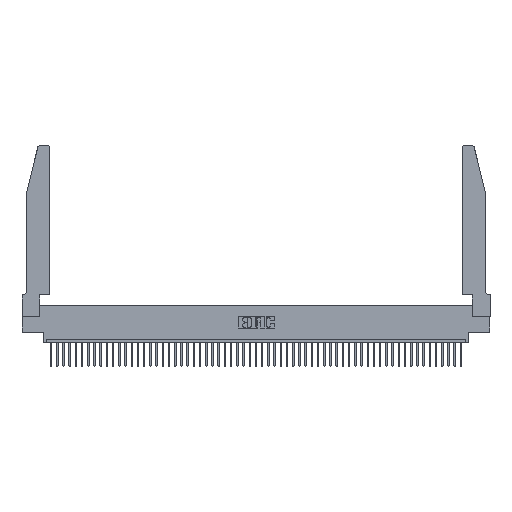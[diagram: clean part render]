
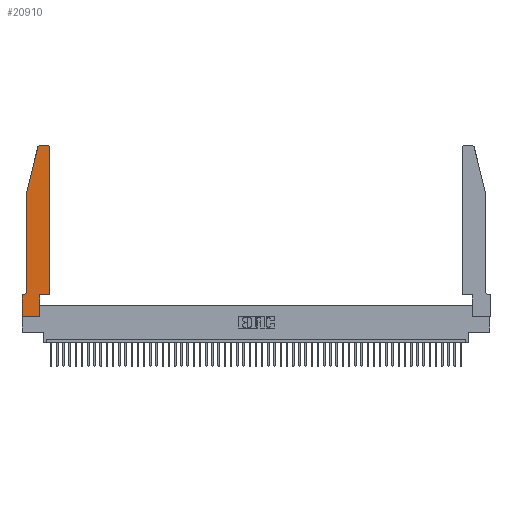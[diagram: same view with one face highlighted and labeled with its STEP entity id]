
A CAD part, top view. The second image highlights one B-rep face of the part: STEP entity #20910.
In plain terms, the highlighted planar face has unit normal (0, 0, 1).
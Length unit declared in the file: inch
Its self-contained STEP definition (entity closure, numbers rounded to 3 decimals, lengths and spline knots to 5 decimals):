
#106 = DIRECTION ( 'NONE',  ( 1., 0., 0. ) ) ;
#670 = CARTESIAN_POINT ( 'NONE',  ( 0.4505, 2.72, 0.37 ) ) ;
#976 = PLANE ( 'NONE',  #9480 ) ;
#1471 = VECTOR ( 'NONE', #15062, 39.37008 ) ;
#2574 = VECTOR ( 'NONE', #45254, 39.37008 ) ;
#3251 = CARTESIAN_POINT ( 'NONE',  ( 0.284, 2.72, 0.37 ) ) ;
#4625 = DIRECTION ( 'NONE',  ( -0.239, -0.971, 0. ) ) ;
#5099 = ORIENTED_EDGE ( 'NONE', *, *, #19223, .T. ) ;
#5565 = ORIENTED_EDGE ( 'NONE', *, *, #37497, .T. ) ;
#5788 = DIRECTION ( 'NONE',  ( -1., 0., 0. ) ) ;
#6047 = CARTESIAN_POINT ( 'NONE',  ( 0.0755, 0.42, 0.37 ) ) ;
#6204 = VERTEX_POINT ( 'NONE', #6047 ) ;
#6361 = VERTEX_POINT ( 'NONE', #27538 ) ;
#7352 = VERTEX_POINT ( 'NONE', #7887 ) ;
#7745 = CARTESIAN_POINT ( 'NONE',  ( 0.25487, 2.72718, 0.37 ) ) ;
#7887 = CARTESIAN_POINT ( 'NONE',  ( 0.0755, 2., 0.37 ) ) ;
#8169 = EDGE_CURVE ( 'NONE', #28078, #36773, #36141, .T. ) ;
#8439 = VECTOR ( 'NONE', #10460, 39.37008 ) ;
#9480 = AXIS2_PLACEMENT_3D ( 'NONE', #13320, #24859, #17191 ) ;
#9971 = DIRECTION ( 'NONE',  ( -1., 0., 0. ) ) ;
#10381 = VECTOR ( 'NONE', #5788, 39.37008 ) ;
#10450 = VERTEX_POINT ( 'NONE', #43552 ) ;
#10460 = DIRECTION ( 'NONE',  ( 0., -1., 0. ) ) ;
#10869 = VERTEX_POINT ( 'NONE', #31786 ) ;
#12723 = VECTOR ( 'NONE', #27065, 39.37008 ) ;
#12754 = CARTESIAN_POINT ( 'NONE',  ( 0.0755, 2., 0.37 ) ) ;
#12926 = CARTESIAN_POINT ( 'NONE',  ( 0.2865, 0.35, 0.37 ) ) ;
#13083 = EDGE_CURVE ( 'NONE', #6204, #28078, #36966, .T. ) ;
#13117 = ORIENTED_EDGE ( 'NONE', *, *, #24074, .T. ) ;
#13320 = CARTESIAN_POINT ( 'NONE',  ( 0., 0.35, 0.37 ) ) ;
#13763 = ORIENTED_EDGE ( 'NONE', *, *, #22768, .T. ) ;
#14435 = CARTESIAN_POINT ( 'NONE',  ( 0.0055, 0.35, 0.37 ) ) ;
#15062 = DIRECTION ( 'NONE',  ( 0., 1., 0. ) ) ;
#15123 = CARTESIAN_POINT ( 'NONE',  ( 0., 0.35, 0.37 ) ) ;
#15197 = LINE ( 'NONE', #22498, #2574 ) ;
#15308 = EDGE_CURVE ( 'NONE', #36773, #22337, #51869, .T. ) ;
#16344 = AXIS2_PLACEMENT_3D ( 'NONE', #20678, #28684, #21019 ) ;
#16410 = CARTESIAN_POINT ( 'NONE',  ( 0.4205, 2.72, 0.37 ) ) ;
#17191 = DIRECTION ( 'NONE',  ( 1., 0., 0. ) ) ;
#18412 = CARTESIAN_POINT ( 'NONE',  ( 0., 0., 0.37 ) ) ;
#19039 = CARTESIAN_POINT ( 'NONE',  ( 0.4505, 0.35, 0.37 ) ) ;
#19223 = EDGE_CURVE ( 'NONE', #10869, #6361, #35547, .T. ) ;
#20595 = EDGE_CURVE ( 'NONE', #28751, #26827, #34877, .T. ) ;
#20678 = CARTESIAN_POINT ( 'NONE',  ( 0.0055, 0.42, 0.37 ) ) ;
#20910 = ADVANCED_FACE ( 'NONE', ( #49197 ), #976, .T. ) ;
#21019 = DIRECTION ( 'NONE',  ( -1., 0., 0. ) ) ;
#21156 = VECTOR ( 'NONE', #4625, 39.37008 ) ;
#22337 = VERTEX_POINT ( 'NONE', #32782 ) ;
#22498 = CARTESIAN_POINT ( 'NONE',  ( 0.4505, 0.35, 0.37 ) ) ;
#22592 = DIRECTION ( 'NONE',  ( 0., -1., 0. ) ) ;
#22768 = EDGE_CURVE ( 'NONE', #7352, #6204, #40495, .T. ) ;
#23132 = VERTEX_POINT ( 'NONE', #670 ) ;
#23422 = LINE ( 'NONE', #19039, #12723 ) ;
#23601 = VECTOR ( 'NONE', #9971, 39.37008 ) ;
#23898 = CARTESIAN_POINT ( 'NONE',  ( 0.0755, 2., 0.37 ) ) ;
#24074 = EDGE_CURVE ( 'NONE', #10450, #23132, #23422, .T. ) ;
#24859 = DIRECTION ( 'NONE',  ( 0., 0., 1. ) ) ;
#24944 = EDGE_CURVE ( 'NONE', #26827, #10450, #15197, .T. ) ;
#25930 = CARTESIAN_POINT ( 'NONE',  ( 0.0755, 0.35, 0.37 ) ) ;
#26827 = VERTEX_POINT ( 'NONE', #12926 ) ;
#27065 = DIRECTION ( 'NONE',  ( 0., 1., 0. ) ) ;
#27412 = DIRECTION ( 'NONE',  ( 0., 0., 1. ) ) ;
#27538 = CARTESIAN_POINT ( 'NONE',  ( 0.284, 2.75, 0.37 ) ) ;
#28068 = CARTESIAN_POINT ( 'NONE',  ( 0., 0., 0.37 ) ) ;
#28078 = VERTEX_POINT ( 'NONE', #14435 ) ;
#28684 = DIRECTION ( 'NONE',  ( 0., 0., -1. ) ) ;
#28751 = VERTEX_POINT ( 'NONE', #45016 ) ;
#29571 = ORIENTED_EDGE ( 'NONE', *, *, #20595, .T. ) ;
#29642 = AXIS2_PLACEMENT_3D ( 'NONE', #16410, #48709, #106 ) ;
#30642 = AXIS2_PLACEMENT_3D ( 'NONE', #3251, #27412, #43130 ) ;
#31010 = EDGE_CURVE ( 'NONE', #6361, #39808, #44079, .T. ) ;
#31786 = CARTESIAN_POINT ( 'NONE',  ( 0.4205, 2.75, 0.37 ) ) ;
#32782 = CARTESIAN_POINT ( 'NONE',  ( 0., 0., 0.37 ) ) ;
#33013 = VECTOR ( 'NONE', #22592, 39.37008 ) ;
#34384 = EDGE_LOOP ( 'NONE', ( #5099, #35303, #5565, #13763, #36234, #51106, #35960, #47236, #29571, #40904, #13117, #43410 ) ) ;
#34877 = LINE ( 'NONE', #43309, #1471 ) ;
#35303 = ORIENTED_EDGE ( 'NONE', *, *, #31010, .T. ) ;
#35547 = LINE ( 'NONE', #49705, #10381 ) ;
#35960 = ORIENTED_EDGE ( 'NONE', *, *, #15308, .T. ) ;
#36141 = LINE ( 'NONE', #25930, #23601 ) ;
#36234 = ORIENTED_EDGE ( 'NONE', *, *, #13083, .T. ) ;
#36773 = VERTEX_POINT ( 'NONE', #15123 ) ;
#36966 = CIRCLE ( 'NONE', #16344, 0.07 ) ;
#37497 = EDGE_CURVE ( 'NONE', #39808, #7352, #40027, .T. ) ;
#39808 = VERTEX_POINT ( 'NONE', #7745 ) ;
#40027 = LINE ( 'NONE', #12754, #21156 ) ;
#40110 = VECTOR ( 'NONE', #44138, 39.37008 ) ;
#40495 = LINE ( 'NONE', #23898, #8439 ) ;
#40904 = ORIENTED_EDGE ( 'NONE', *, *, #24944, .T. ) ;
#43130 = DIRECTION ( 'NONE',  ( 1., 0., 0. ) ) ;
#43309 = CARTESIAN_POINT ( 'NONE',  ( 0.2865, 0.35, 0.37 ) ) ;
#43410 = ORIENTED_EDGE ( 'NONE', *, *, #48120, .T. ) ;
#43552 = CARTESIAN_POINT ( 'NONE',  ( 0.4505, 0.35, 0.37 ) ) ;
#44079 = CIRCLE ( 'NONE', #30642, 0.03 ) ;
#44138 = DIRECTION ( 'NONE',  ( 1., 0., 0. ) ) ;
#45016 = CARTESIAN_POINT ( 'NONE',  ( 0.2865, 0., 0.37 ) ) ;
#45254 = DIRECTION ( 'NONE',  ( 1., 0., 0. ) ) ;
#47236 = ORIENTED_EDGE ( 'NONE', *, *, #49758, .T. ) ;
#48120 = EDGE_CURVE ( 'NONE', #23132, #10869, #50348, .T. ) ;
#48709 = DIRECTION ( 'NONE',  ( 0., 0., 1. ) ) ;
#49197 = FACE_OUTER_BOUND ( 'NONE', #34384, .T. ) ;
#49705 = CARTESIAN_POINT ( 'NONE',  ( 0.2605, 2.75, 0.37 ) ) ;
#49758 = EDGE_CURVE ( 'NONE', #22337, #28751, #50790, .T. ) ;
#50348 = CIRCLE ( 'NONE', #29642, 0.03 ) ;
#50790 = LINE ( 'NONE', #28068, #40110 ) ;
#51106 = ORIENTED_EDGE ( 'NONE', *, *, #8169, .T. ) ;
#51869 = LINE ( 'NONE', #18412, #33013 ) ;
